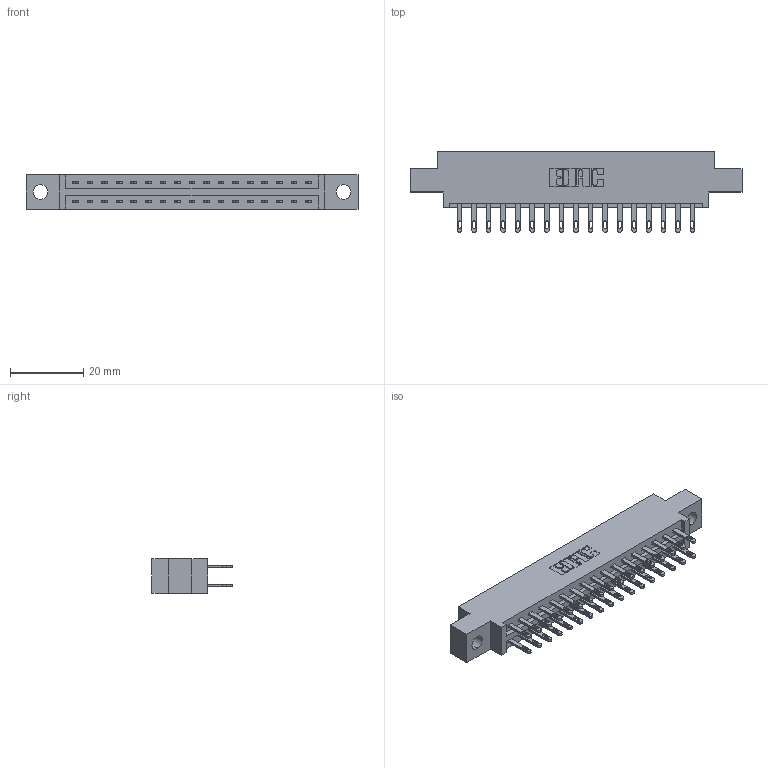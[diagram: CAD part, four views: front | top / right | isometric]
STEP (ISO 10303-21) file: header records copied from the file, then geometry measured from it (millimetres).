
FILE_DESCRIPTION (( 'STEP AP203' ), '1' );
FILE_NAME ('337-034-500-804.STEP', '2018-08-07T09:59:10', ( '' ), ( '' ), 'SwSTEP 2.0', 'SolidWorks 2016', '' );
FILE_SCHEMA (( 'CONFIG_CONTROL_DESIGN' ));
Length unit declared in the file: inch
Products named in the file (3): 337-034-500-804; 337 Part_0.170 Offset - 0.156 Dia-TH; 345-292-001_345-293-100
Assembly tree (35 placements, depth 2):
  337-034-500-804
    337 Part_0.170 Offset - 0.156 Dia-TH
    345-292-001_345-293-100  x34
Bounding box: 90.37 x 21.85 x 9.4 mm (x, y, z)
Volume: 9090 mm3; surface area: 10315.9 mm2
Topology: 35 solids, 35 shells, 1818 faces, 5525 edges, 3682 vertices
Faces by surface type: plane 1162, cylinder 656
Entity records: 16479 total; most frequent: CARTESIAN_POINT 2798, ORIENTED_EDGE 2734, DIRECTION 2427, EDGE_CURVE 1367, VECTOR 1235, LINE 1235, VERTEX_POINT 910, AXIS2_PLACEMENT_3D 596
